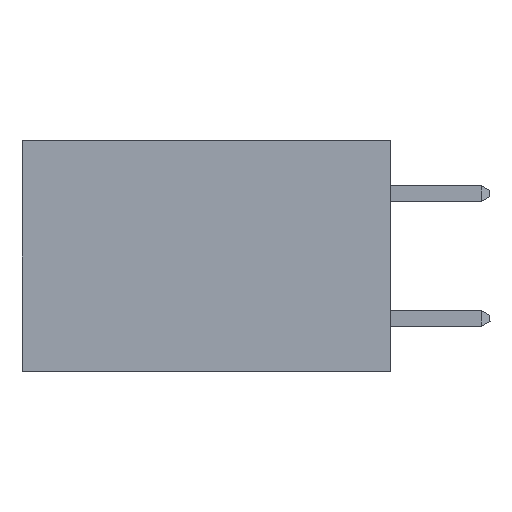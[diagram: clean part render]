
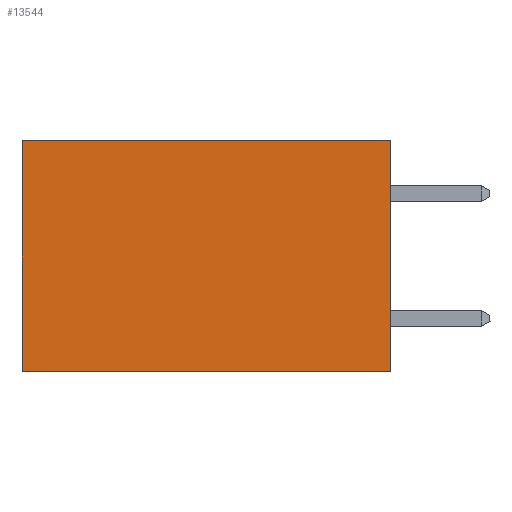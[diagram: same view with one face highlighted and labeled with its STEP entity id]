
A CAD part, left-side view. The second image highlights one B-rep face of the part: STEP entity #13544.
In plain terms, the highlighted planar face has unit normal (-1, 0, 0).
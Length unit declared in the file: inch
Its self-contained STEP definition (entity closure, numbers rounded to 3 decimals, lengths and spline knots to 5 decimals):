
#432 = VECTOR ( 'NONE', #18822, 39.37008 ) ;
#1162 = EDGE_CURVE ( 'NONE', #16985, #16510, #4627, .T. ) ;
#1297 = VECTOR ( 'NONE', #21508, 39.37008 ) ;
#2215 = ORIENTED_EDGE ( 'NONE', *, *, #3557, .F. ) ;
#2436 = ORIENTED_EDGE ( 'NONE', *, *, #10440, .T. ) ;
#2632 = DIRECTION ( 'NONE',  ( 0., 1., 0. ) ) ;
#3069 = CARTESIAN_POINT ( 'NONE',  ( 0.277, 0.59, 0. ) ) ;
#3317 = ORIENTED_EDGE ( 'NONE', *, *, #5266, .T. ) ;
#3452 = VERTEX_POINT ( 'NONE', #3069 ) ;
#3557 = EDGE_CURVE ( 'NONE', #16510, #15480, #3907, .T. ) ;
#3907 = LINE ( 'NONE', #10953, #8128 ) ;
#4627 = LINE ( 'NONE', #20530, #432 ) ;
#5266 = EDGE_CURVE ( 'NONE', #16985, #3452, #10217, .T. ) ;
#5959 = CARTESIAN_POINT ( 'NONE',  ( 0.277, 0.59, -0.37 ) ) ;
#6344 = CARTESIAN_POINT ( 'NONE',  ( 0.277, 0., -0.37 ) ) ;
#7162 = LINE ( 'NONE', #5959, #15353 ) ;
#8128 = VECTOR ( 'NONE', #2632, 39.37008 ) ;
#9703 = CARTESIAN_POINT ( 'NONE',  ( 0.277, 0.59, -0.37 ) ) ;
#9910 = DIRECTION ( 'NONE',  ( 0., 0., -1. ) ) ;
#10217 = LINE ( 'NONE', #21645, #1297 ) ;
#10440 = EDGE_CURVE ( 'NONE', #3452, #15480, #7162, .T. ) ;
#10953 = CARTESIAN_POINT ( 'NONE',  ( 0.277, 0., -0.37 ) ) ;
#11208 = DIRECTION ( 'NONE',  ( 0., 0., -1. ) ) ;
#11786 = CARTESIAN_POINT ( 'NONE',  ( 0.277, 0., 0. ) ) ;
#12038 = CARTESIAN_POINT ( 'NONE',  ( 0.277, 0., -0.37 ) ) ;
#12412 = EDGE_LOOP ( 'NONE', ( #2436, #2215, #16486, #3317 ) ) ;
#13544 = ADVANCED_FACE ( 'NONE', ( #21040 ), #16774, .F. ) ;
#15353 = VECTOR ( 'NONE', #11208, 39.37008 ) ;
#15480 = VERTEX_POINT ( 'NONE', #9703 ) ;
#16024 = AXIS2_PLACEMENT_3D ( 'NONE', #6344, #20153, #9910 ) ;
#16486 = ORIENTED_EDGE ( 'NONE', *, *, #1162, .F. ) ;
#16510 = VERTEX_POINT ( 'NONE', #12038 ) ;
#16774 = PLANE ( 'NONE',  #16024 ) ;
#16985 = VERTEX_POINT ( 'NONE', #11786 ) ;
#18822 = DIRECTION ( 'NONE',  ( 0., 0., -1. ) ) ;
#20153 = DIRECTION ( 'NONE',  ( 1., 0., 0. ) ) ;
#20530 = CARTESIAN_POINT ( 'NONE',  ( 0.277, 0., -0.37 ) ) ;
#21040 = FACE_OUTER_BOUND ( 'NONE', #12412, .T. ) ;
#21508 = DIRECTION ( 'NONE',  ( 0., 1., 0. ) ) ;
#21645 = CARTESIAN_POINT ( 'NONE',  ( 0.277, 0., 0. ) ) ;
